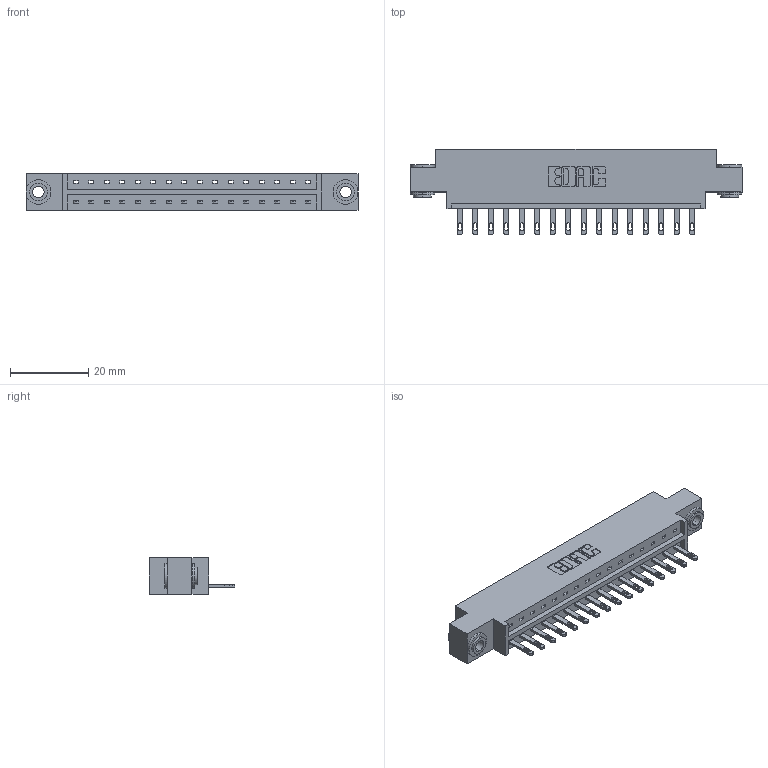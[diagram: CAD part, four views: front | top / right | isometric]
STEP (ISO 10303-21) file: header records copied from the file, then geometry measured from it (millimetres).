
FILE_DESCRIPTION (( 'STEP AP203' ), '1' );
FILE_NAME ('333-016-500-603.STEP', '2018-08-01T11:15:20', ( '' ), ( '' ), 'SwSTEP 2.0', 'SolidWorks 2016', '' );
FILE_SCHEMA (( 'CONFIG_CONTROL_DESIGN' ));
Length unit declared in the file: inch
Products named in the file (4): 345-250-002_345-250-002-102; 333-016-500-603; 333 Part_Offset - .156 Dia - TH; 345-292-001_345-293-100
Assembly tree (19 placements, depth 2):
  333-016-500-603
    333 Part_Offset - .156 Dia - TH
    345-292-001_345-293-100  x16
    345-250-002_345-250-002-102  x2
Bounding box: 84.94 x 21.85 x 9.4 mm (x, y, z)
Volume: 8125 mm3; surface area: 9085.4 mm2
Topology: 19 solids, 19 shells, 1020 faces, 3087 edges, 2054 vertices
Faces by surface type: plane 660, cylinder 352, cone 8
Entity records: 13856 total; most frequent: CARTESIAN_POINT 2373, ORIENTED_EDGE 2318, DIRECTION 2089, EDGE_CURVE 1159, LINE 1003, VECTOR 1003, VERTEX_POINT 770, AXIS2_PLACEMENT_3D 543
